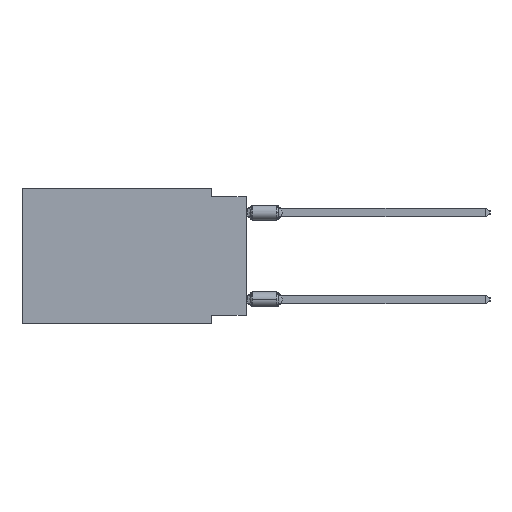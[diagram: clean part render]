
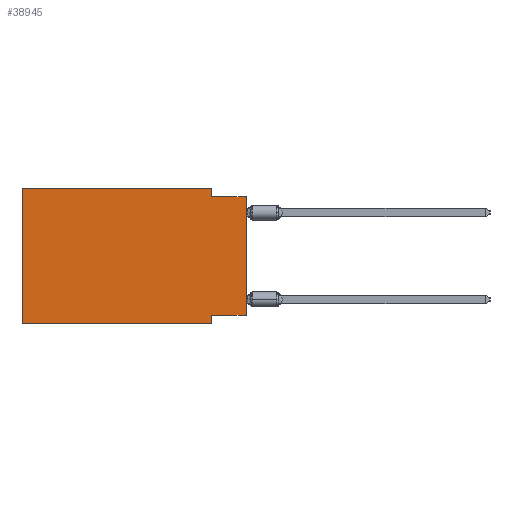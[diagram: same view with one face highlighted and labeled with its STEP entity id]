
A CAD part, left-side view. The second image highlights one B-rep face of the part: STEP entity #38945.
In plain terms, the highlighted planar face has unit normal (-1, 0, 0).
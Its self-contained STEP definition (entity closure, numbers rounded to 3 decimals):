
#36 = VECTOR ( 'NONE', #30853, 1000. ) ;
#206 = LINE ( 'NONE', #2807, #36 ) ;
#1327 = VERTEX_POINT ( 'NONE', #39295 ) ;
#2249 = VECTOR ( 'NONE', #13282, 1000. ) ;
#2275 = AXIS2_PLACEMENT_3D ( 'NONE', #33499, #34094, #39512 ) ;
#2807 = CARTESIAN_POINT ( 'NONE',  ( 0., 0., -9.271 ) ) ;
#7145 = ORIENTED_EDGE ( 'NONE', *, *, #10960, .T. ) ;
#7454 = CARTESIAN_POINT ( 'NONE',  ( 0., 0., 0. ) ) ;
#7528 = LINE ( 'NONE', #37961, #17479 ) ;
#7649 = DIRECTION ( 'NONE',  ( 0., 0., 1. ) ) ;
#8097 = EDGE_CURVE ( 'NONE', #15018, #31473, #28274, .T. ) ;
#9106 = EDGE_CURVE ( 'NONE', #31473, #19025, #35912, .T. ) ;
#10062 = CARTESIAN_POINT ( 'NONE',  ( 0., 2.54, 0. ) ) ;
#10457 = VERTEX_POINT ( 'NONE', #26491 ) ;
#10460 = LINE ( 'NONE', #7454, #29083 ) ;
#10960 = EDGE_CURVE ( 'NONE', #32244, #19025, #10460, .T. ) ;
#12048 = EDGE_LOOP ( 'NONE', ( #7145, #17136, #25692, #14439, #35415, #35054, #34479, #20196 ) ) ;
#13282 = DIRECTION ( 'NONE',  ( 0., 0., -1. ) ) ;
#14304 = DIRECTION ( 'NONE',  ( 0., -1., 0. ) ) ;
#14439 = ORIENTED_EDGE ( 'NONE', *, *, #26919, .F. ) ;
#14977 = LINE ( 'NONE', #36408, #32640 ) ;
#15018 = VERTEX_POINT ( 'NONE', #20794 ) ;
#15238 = CARTESIAN_POINT ( 'NONE',  ( 0., 16.383, 0. ) ) ;
#15650 = CARTESIAN_POINT ( 'NONE',  ( 0., 0., -9.271 ) ) ;
#16724 = DIRECTION ( 'NONE',  ( 0., 0., -1. ) ) ;
#17136 = ORIENTED_EDGE ( 'NONE', *, *, #9106, .F. ) ;
#17479 = VECTOR ( 'NONE', #16724, 1000. ) ;
#18362 = VERTEX_POINT ( 'NONE', #27775 ) ;
#18436 = LINE ( 'NONE', #15238, #28166 ) ;
#19025 = VERTEX_POINT ( 'NONE', #24228 ) ;
#19531 = EDGE_CURVE ( 'NONE', #35934, #10457, #14977, .T. ) ;
#19685 = CARTESIAN_POINT ( 'NONE',  ( 0., 16.383, 0. ) ) ;
#20196 = ORIENTED_EDGE ( 'NONE', *, *, #34446, .F. ) ;
#20794 = CARTESIAN_POINT ( 'NONE',  ( 0., 2.54, 0. ) ) ;
#21494 = FACE_OUTER_BOUND ( 'NONE', #12048, .T. ) ;
#22644 = VECTOR ( 'NONE', #37913, 1000. ) ;
#22738 = CARTESIAN_POINT ( 'NONE',  ( 0., 2.54, -0.635 ) ) ;
#22887 = LINE ( 'NONE', #19685, #22644 ) ;
#23348 = EDGE_CURVE ( 'NONE', #1327, #10457, #7528, .T. ) ;
#24228 = CARTESIAN_POINT ( 'NONE',  ( 0., 0., -0.635 ) ) ;
#25692 = ORIENTED_EDGE ( 'NONE', *, *, #8097, .F. ) ;
#26312 = CARTESIAN_POINT ( 'NONE',  ( 0., 0., -0.635 ) ) ;
#26491 = CARTESIAN_POINT ( 'NONE',  ( 0., 2.54, -9.906 ) ) ;
#26919 = EDGE_CURVE ( 'NONE', #18362, #15018, #22887, .T. ) ;
#27775 = CARTESIAN_POINT ( 'NONE',  ( 0., 16.383, 0. ) ) ;
#28166 = VECTOR ( 'NONE', #30653, 1000. ) ;
#28274 = LINE ( 'NONE', #10062, #2249 ) ;
#29083 = VECTOR ( 'NONE', #7649, 1000. ) ;
#29596 = DIRECTION ( 'NONE',  ( 0., -1., 0. ) ) ;
#30653 = DIRECTION ( 'NONE',  ( 0., 0., 1. ) ) ;
#30853 = DIRECTION ( 'NONE',  ( 0., 1., 0. ) ) ;
#31473 = VERTEX_POINT ( 'NONE', #22738 ) ;
#32244 = VERTEX_POINT ( 'NONE', #15650 ) ;
#32640 = VECTOR ( 'NONE', #29596, 1000. ) ;
#33499 = CARTESIAN_POINT ( 'NONE',  ( 0., 16.383, 0. ) ) ;
#33898 = PLANE ( 'NONE',  #2275 ) ;
#34094 = DIRECTION ( 'NONE',  ( 1., 0., 0. ) ) ;
#34446 = EDGE_CURVE ( 'NONE', #32244, #1327, #206, .T. ) ;
#34463 = EDGE_CURVE ( 'NONE', #35934, #18362, #18436, .T. ) ;
#34479 = ORIENTED_EDGE ( 'NONE', *, *, #23348, .F. ) ;
#34848 = CARTESIAN_POINT ( 'NONE',  ( 0., 16.383, -9.906 ) ) ;
#35054 = ORIENTED_EDGE ( 'NONE', *, *, #19531, .T. ) ;
#35415 = ORIENTED_EDGE ( 'NONE', *, *, #34463, .F. ) ;
#35912 = LINE ( 'NONE', #26312, #36852 ) ;
#35934 = VERTEX_POINT ( 'NONE', #34848 ) ;
#36408 = CARTESIAN_POINT ( 'NONE',  ( 0., 16.383, -9.906 ) ) ;
#36852 = VECTOR ( 'NONE', #14304, 1000. ) ;
#37913 = DIRECTION ( 'NONE',  ( 0., -1., 0. ) ) ;
#37961 = CARTESIAN_POINT ( 'NONE',  ( 0., 2.54, -9.906 ) ) ;
#38945 = ADVANCED_FACE ( 'NONE', ( #21494 ), #33898, .F. ) ;
#39295 = CARTESIAN_POINT ( 'NONE',  ( 0., 2.54, -9.271 ) ) ;
#39512 = DIRECTION ( 'NONE',  ( 0., 0., -1. ) ) ;
